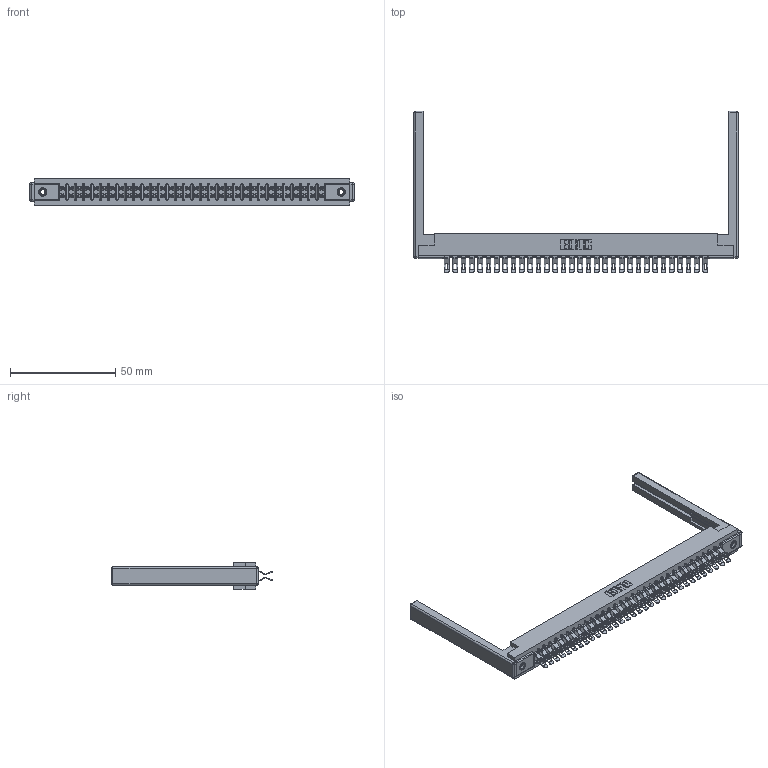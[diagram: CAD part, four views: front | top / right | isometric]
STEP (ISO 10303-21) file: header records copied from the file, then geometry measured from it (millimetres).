
FILE_DESCRIPTION (( 'STEP AP203' ), '1' );
FILE_NAME ('307-064-555-268.STEP', '2019-09-06T16:58:16', ( '' ), ( '' ), 'SwSTEP 2.0', 'SolidWorks 2016', '' );
FILE_SCHEMA (( 'CONFIG_CONTROL_DESIGN' ));
Length unit declared in the file: inch
Products named in the file (5): 307-220-068; 307 Part_.156 Dia Mounting Holes; 345-250-001_345-250-001-102; 307-290-001_555; 307-064-555-268
Assembly tree (69 placements, depth 2):
  307-064-555-268
    307 Part_.156 Dia Mounting Holes
    307-290-001_555  x64
    307-220-068  x2
    345-250-001_345-250-001-102  x2
Bounding box: 154.23 x 76.71 x 12.7 mm (x, y, z)
Volume: 20900.8 mm3; surface area: 25051.9 mm2
Topology: 69 solids, 69 shells, 4209 faces, 12297 edges, 8002 vertices
Faces by surface type: plane 2334, cylinder 1785, sphere 74, cone 12, torus 4
Entity records: 32986 total; most frequent: CARTESIAN_POINT 5381, ORIENTED_EDGE 5326, DIRECTION 5297, EDGE_CURVE 2663, VECTOR 2025, LINE 2025, VERTEX_POINT 1720, AXIS2_PLACEMENT_3D 1636
